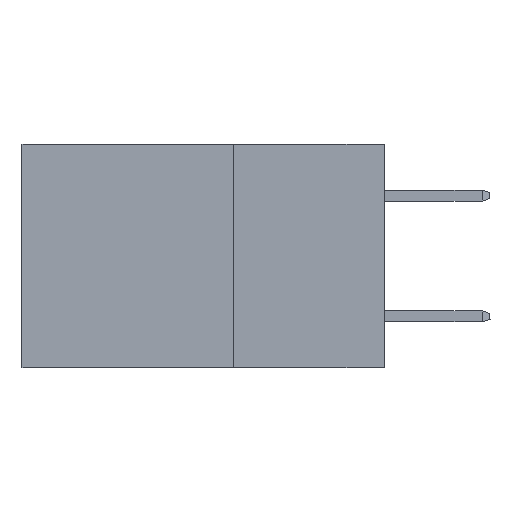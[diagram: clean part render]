
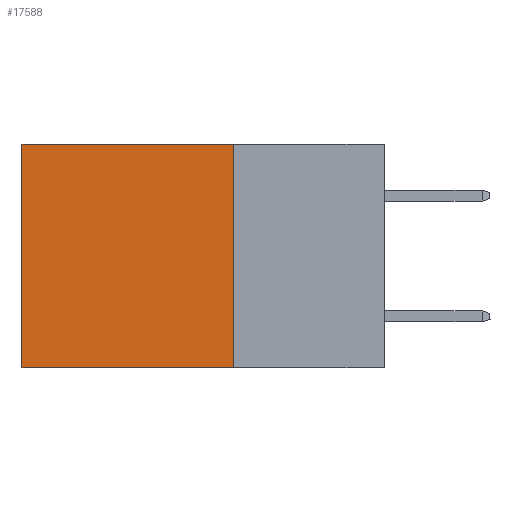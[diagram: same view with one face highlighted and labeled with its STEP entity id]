
A CAD part, left-side view. The second image highlights one B-rep face of the part: STEP entity #17588.
In plain terms, the highlighted planar face has unit normal (-1, 0, 0).
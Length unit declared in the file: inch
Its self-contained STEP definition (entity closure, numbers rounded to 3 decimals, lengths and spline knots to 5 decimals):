
#335 = VERTEX_POINT ( 'NONE', #5099 ) ;
#360 = ORIENTED_EDGE ( 'NONE', *, *, #11116, .T. ) ;
#1206 = ORIENTED_EDGE ( 'NONE', *, *, #9541, .F. ) ;
#1715 = VERTEX_POINT ( 'NONE', #13055 ) ;
#2668 = VERTEX_POINT ( 'NONE', #10246 ) ;
#2795 = AXIS2_PLACEMENT_3D ( 'NONE', #13119, #14521, #5916 ) ;
#3022 = VECTOR ( 'NONE', #15507, 39.37008 ) ;
#3060 = CARTESIAN_POINT ( 'NONE',  ( 0.2615, 0.25, 0. ) ) ;
#3117 = VECTOR ( 'NONE', #15389, 39.37008 ) ;
#5002 = CARTESIAN_POINT ( 'NONE',  ( 0.2615, 0.25, -0.37 ) ) ;
#5099 = CARTESIAN_POINT ( 'NONE',  ( 0.2615, 0.6, -0.37 ) ) ;
#5567 = EDGE_CURVE ( 'NONE', #1715, #335, #10746, .T. ) ;
#5916 = DIRECTION ( 'NONE',  ( 0., 0., -1. ) ) ;
#6018 = DIRECTION ( 'NONE',  ( 0., 1., 0. ) ) ;
#6042 = ORIENTED_EDGE ( 'NONE', *, *, #8259, .F. ) ;
#6485 = DIRECTION ( 'NONE',  ( 0., 0., -1. ) ) ;
#7054 = VECTOR ( 'NONE', #6485, 39.37008 ) ;
#7299 = PLANE ( 'NONE',  #2795 ) ;
#8198 = VERTEX_POINT ( 'NONE', #13527 ) ;
#8259 = EDGE_CURVE ( 'NONE', #8198, #2668, #18433, .T. ) ;
#8878 = CARTESIAN_POINT ( 'NONE',  ( 0.2615, 0.25, -0.37 ) ) ;
#9541 = EDGE_CURVE ( 'NONE', #2668, #335, #18373, .T. ) ;
#10246 = CARTESIAN_POINT ( 'NONE',  ( 0.2615, 0.25, -0.37 ) ) ;
#10746 = LINE ( 'NONE', #13131, #3022 ) ;
#10951 = FACE_OUTER_BOUND ( 'NONE', #11470, .T. ) ;
#11116 = EDGE_CURVE ( 'NONE', #8198, #1715, #14108, .T. ) ;
#11164 = ORIENTED_EDGE ( 'NONE', *, *, #5567, .T. ) ;
#11470 = EDGE_LOOP ( 'NONE', ( #11164, #1206, #6042, #360 ) ) ;
#13055 = CARTESIAN_POINT ( 'NONE',  ( 0.2615, 0.6, 0. ) ) ;
#13119 = CARTESIAN_POINT ( 'NONE',  ( 0.2615, 0.25, -0.37 ) ) ;
#13131 = CARTESIAN_POINT ( 'NONE',  ( 0.2615, 0.6, -0.37 ) ) ;
#13527 = CARTESIAN_POINT ( 'NONE',  ( 0.2615, 0.25, 0. ) ) ;
#13683 = VECTOR ( 'NONE', #6018, 39.37008 ) ;
#14108 = LINE ( 'NONE', #3060, #13683 ) ;
#14521 = DIRECTION ( 'NONE',  ( 1., 0., 0. ) ) ;
#15389 = DIRECTION ( 'NONE',  ( 0., 1., 0. ) ) ;
#15507 = DIRECTION ( 'NONE',  ( 0., 0., -1. ) ) ;
#17588 = ADVANCED_FACE ( 'NONE', ( #10951 ), #7299, .F. ) ;
#18373 = LINE ( 'NONE', #8878, #3117 ) ;
#18433 = LINE ( 'NONE', #5002, #7054 ) ;
